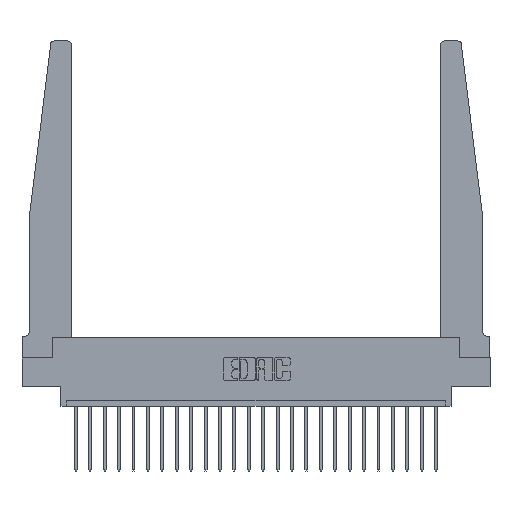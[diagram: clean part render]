
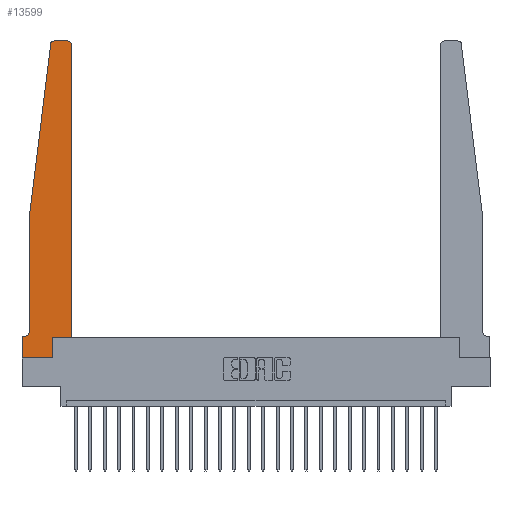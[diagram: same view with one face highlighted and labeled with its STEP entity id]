
A CAD part, top view. The second image highlights one B-rep face of the part: STEP entity #13599.
In plain terms, the highlighted planar face has unit normal (0, 0, 1).
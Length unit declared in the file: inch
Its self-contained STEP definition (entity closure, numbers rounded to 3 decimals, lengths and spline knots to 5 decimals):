
#102 = DIRECTION ( 'NONE',  ( 0., 0., 1. ) ) ;
#465 = VECTOR ( 'NONE', #18315, 39.37008 ) ;
#664 = DIRECTION ( 'NONE',  ( 1., 0., 0. ) ) ;
#704 = VECTOR ( 'NONE', #14985, 39.37008 ) ;
#945 = ORIENTED_EDGE ( 'NONE', *, *, #2882, .T. ) ;
#1028 = CARTESIAN_POINT ( 'NONE',  ( 0., 0., 0.37 ) ) ;
#1176 = DIRECTION ( 'NONE',  ( 1., 0., 0. ) ) ;
#1450 = DIRECTION ( 'NONE',  ( 0., 0., 1. ) ) ;
#1455 = VECTOR ( 'NONE', #20403, 39.37008 ) ;
#2353 = CARTESIAN_POINT ( 'NONE',  ( 0.2605, 0.18, 0.37 ) ) ;
#2691 = ORIENTED_EDGE ( 'NONE', *, *, #22400, .T. ) ;
#2700 = CARTESIAN_POINT ( 'NONE',  ( 0.2605, 0.18, 0.37 ) ) ;
#2881 = CARTESIAN_POINT ( 'NONE',  ( 0.065, 1.25, 0.37 ) ) ;
#2882 = EDGE_CURVE ( 'NONE', #15678, #20808, #15006, .T. ) ;
#3110 = ORIENTED_EDGE ( 'NONE', *, *, #17008, .T. ) ;
#3128 = CARTESIAN_POINT ( 'NONE',  ( 0.395, 2.72, 0.37 ) ) ;
#3277 = VERTEX_POINT ( 'NONE', #22163 ) ;
#3687 = CIRCLE ( 'NONE', #23165, 0.03 ) ;
#3757 = CARTESIAN_POINT ( 'NONE',  ( 0.425, 0.18, 0.37 ) ) ;
#4080 = CARTESIAN_POINT ( 'NONE',  ( 0.27653, 2.75, 0.37 ) ) ;
#4088 = CARTESIAN_POINT ( 'NONE',  ( 0.065, 0.1875, 0.37 ) ) ;
#4188 = ORIENTED_EDGE ( 'NONE', *, *, #15517, .T. ) ;
#5037 = DIRECTION ( 'NONE',  ( 1., 0., 0. ) ) ;
#5358 = ORIENTED_EDGE ( 'NONE', *, *, #16912, .T. ) ;
#5534 = CARTESIAN_POINT ( 'NONE',  ( 0.015, 0.2375, 0.37 ) ) ;
#5869 = EDGE_CURVE ( 'NONE', #22154, #21163, #11412, .T. ) ;
#5933 = CARTESIAN_POINT ( 'NONE',  ( 0.065, 1.25, 0.37 ) ) ;
#6026 = DIRECTION ( 'NONE',  ( 0., 1., 0. ) ) ;
#7440 = VERTEX_POINT ( 'NONE', #4080 ) ;
#7572 = LINE ( 'NONE', #18577, #704 ) ;
#8058 = VECTOR ( 'NONE', #18660, 39.37008 ) ;
#9169 = PLANE ( 'NONE',  #17375 ) ;
#9235 = LINE ( 'NONE', #14605, #465 ) ;
#9390 = VERTEX_POINT ( 'NONE', #11305 ) ;
#9510 = VECTOR ( 'NONE', #12975, 39.37008 ) ;
#9662 = ORIENTED_EDGE ( 'NONE', *, *, #15091, .T. ) ;
#9745 = FACE_OUTER_BOUND ( 'NONE', #10450, .T. ) ;
#9855 = CARTESIAN_POINT ( 'NONE',  ( 0.25, 2.75, 0.37 ) ) ;
#9980 = VERTEX_POINT ( 'NONE', #14092 ) ;
#10450 = EDGE_LOOP ( 'NONE', ( #9662, #5358, #945, #13789, #4188, #12576, #21225, #2691, #20040, #17362, #18350, #3110 ) ) ;
#10852 = EDGE_CURVE ( 'NONE', #13059, #10998, #17046, .T. ) ;
#10906 = DIRECTION ( 'NONE',  ( 0., 0., -1. ) ) ;
#10998 = VERTEX_POINT ( 'NONE', #2700 ) ;
#11105 = VECTOR ( 'NONE', #6026, 39.37008 ) ;
#11305 = CARTESIAN_POINT ( 'NONE',  ( 0.065, 0.2375, 0.37 ) ) ;
#11412 = LINE ( 'NONE', #3757, #11105 ) ;
#11886 = LINE ( 'NONE', #9855, #19091 ) ;
#12576 = ORIENTED_EDGE ( 'NONE', *, *, #21978, .T. ) ;
#12975 = DIRECTION ( 'NONE',  ( 0., 1., 0. ) ) ;
#13059 = VERTEX_POINT ( 'NONE', #23095 ) ;
#13170 = LINE ( 'NONE', #4088, #8058 ) ;
#13440 = DIRECTION ( 'NONE',  ( -1., 0., 0. ) ) ;
#13472 = VECTOR ( 'NONE', #22358, 39.37008 ) ;
#13599 = ADVANCED_FACE ( 'NONE', ( #9745 ), #9169, .T. ) ;
#13789 = ORIENTED_EDGE ( 'NONE', *, *, #18275, .T. ) ;
#14092 = CARTESIAN_POINT ( 'NONE',  ( 0.015, 0.1875, 0.37 ) ) ;
#14605 = CARTESIAN_POINT ( 'NONE',  ( 0.425, 0.18, 0.37 ) ) ;
#14724 = CARTESIAN_POINT ( 'NONE',  ( 0., 0.1875, 0.37 ) ) ;
#14841 = DIRECTION ( 'NONE',  ( -1., 0., 0. ) ) ;
#14985 = DIRECTION ( 'NONE',  ( 0., -1., 0. ) ) ;
#15006 = LINE ( 'NONE', #5933, #1455 ) ;
#15091 = EDGE_CURVE ( 'NONE', #3277, #7440, #11886, .T. ) ;
#15403 = CARTESIAN_POINT ( 'NONE',  ( 0.425, 2.72, 0.37 ) ) ;
#15435 = EDGE_CURVE ( 'NONE', #10998, #22154, #9235, .T. ) ;
#15517 = EDGE_CURVE ( 'NONE', #9390, #9980, #17693, .T. ) ;
#15678 = VERTEX_POINT ( 'NONE', #21538 ) ;
#15749 = LINE ( 'NONE', #17543, #16462 ) ;
#16460 = CARTESIAN_POINT ( 'NONE',  ( 0., 0.1875, 0.37 ) ) ;
#16462 = VECTOR ( 'NONE', #1176, 39.37008 ) ;
#16654 = AXIS2_PLACEMENT_3D ( 'NONE', #18906, #18790, #19020 ) ;
#16689 = VERTEX_POINT ( 'NONE', #14724 ) ;
#16912 = EDGE_CURVE ( 'NONE', #7440, #15678, #19696, .T. ) ;
#17008 = EDGE_CURVE ( 'NONE', #21163, #3277, #3687, .T. ) ;
#17046 = LINE ( 'NONE', #2353, #9510 ) ;
#17069 = LINE ( 'NONE', #22467, #13472 ) ;
#17362 = ORIENTED_EDGE ( 'NONE', *, *, #15435, .T. ) ;
#17375 = AXIS2_PLACEMENT_3D ( 'NONE', #16460, #102, #664 ) ;
#17543 = CARTESIAN_POINT ( 'NONE',  ( 0., 0., 0.37 ) ) ;
#17693 = CIRCLE ( 'NONE', #20391, 0.05 ) ;
#18275 = EDGE_CURVE ( 'NONE', #20808, #9390, #17069, .T. ) ;
#18315 = DIRECTION ( 'NONE',  ( 1., 0., 0. ) ) ;
#18350 = ORIENTED_EDGE ( 'NONE', *, *, #5869, .T. ) ;
#18577 = CARTESIAN_POINT ( 'NONE',  ( 0., 0., 0.37 ) ) ;
#18660 = DIRECTION ( 'NONE',  ( -1., 0., 0. ) ) ;
#18790 = DIRECTION ( 'NONE',  ( 0., 0., 1. ) ) ;
#18847 = VERTEX_POINT ( 'NONE', #1028 ) ;
#18906 = CARTESIAN_POINT ( 'NONE',  ( 0.27653, 2.72, 0.37 ) ) ;
#19020 = DIRECTION ( 'NONE',  ( 1., 0., 0. ) ) ;
#19091 = VECTOR ( 'NONE', #13440, 39.37008 ) ;
#19696 = CIRCLE ( 'NONE', #16654, 0.03 ) ;
#20040 = ORIENTED_EDGE ( 'NONE', *, *, #10852, .T. ) ;
#20194 = EDGE_CURVE ( 'NONE', #16689, #18847, #7572, .T. ) ;
#20391 = AXIS2_PLACEMENT_3D ( 'NONE', #5534, #10906, #14841 ) ;
#20403 = DIRECTION ( 'NONE',  ( -0.122, -0.992, 0. ) ) ;
#20808 = VERTEX_POINT ( 'NONE', #2881 ) ;
#21163 = VERTEX_POINT ( 'NONE', #15403 ) ;
#21225 = ORIENTED_EDGE ( 'NONE', *, *, #20194, .T. ) ;
#21538 = CARTESIAN_POINT ( 'NONE',  ( 0.24675, 2.72367, 0.37 ) ) ;
#21978 = EDGE_CURVE ( 'NONE', #9980, #16689, #13170, .T. ) ;
#22154 = VERTEX_POINT ( 'NONE', #22233 ) ;
#22163 = CARTESIAN_POINT ( 'NONE',  ( 0.395, 2.75, 0.37 ) ) ;
#22233 = CARTESIAN_POINT ( 'NONE',  ( 0.425, 0.18, 0.37 ) ) ;
#22358 = DIRECTION ( 'NONE',  ( 0., -1., 0. ) ) ;
#22400 = EDGE_CURVE ( 'NONE', #18847, #13059, #15749, .T. ) ;
#22467 = CARTESIAN_POINT ( 'NONE',  ( 0.065, 1.25, 0.37 ) ) ;
#23095 = CARTESIAN_POINT ( 'NONE',  ( 0.2605, 0., 0.37 ) ) ;
#23165 = AXIS2_PLACEMENT_3D ( 'NONE', #3128, #1450, #5037 ) ;
